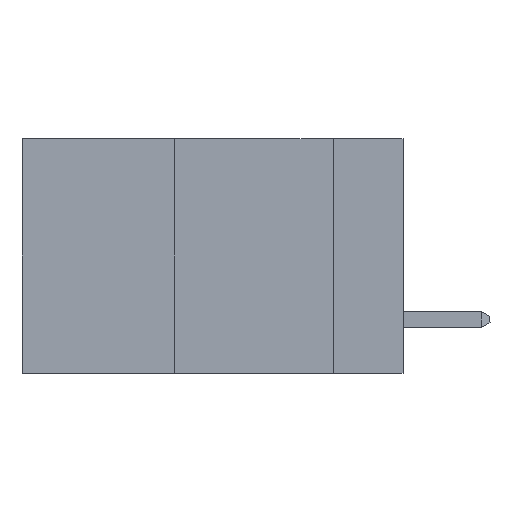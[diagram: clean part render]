
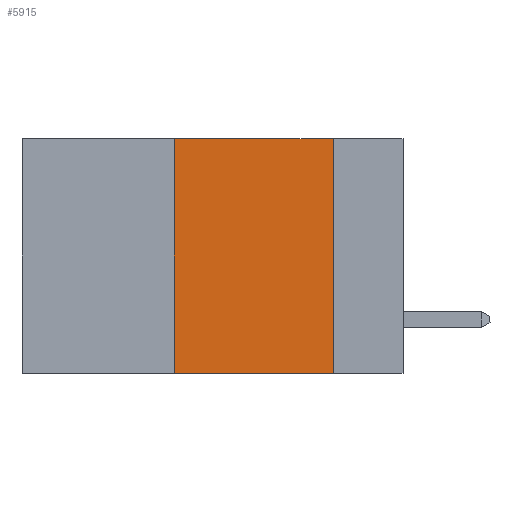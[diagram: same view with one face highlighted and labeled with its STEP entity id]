
A CAD part, left-side view. The second image highlights one B-rep face of the part: STEP entity #5915.
In plain terms, the highlighted planar face has unit normal (-1, 0, 0).
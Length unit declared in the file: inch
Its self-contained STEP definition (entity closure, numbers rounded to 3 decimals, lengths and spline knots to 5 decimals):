
#116 = DIRECTION ( 'NONE',  ( 1., 0., 0. ) ) ;
#634 = DIRECTION ( 'NONE',  ( 0., -1., 0. ) ) ;
#686 = VERTEX_POINT ( 'NONE', #8401 ) ;
#2073 = CARTESIAN_POINT ( 'NONE',  ( 0., 0.36, 0. ) ) ;
#2184 = EDGE_LOOP ( 'NONE', ( #16346, #13541, #3752, #4195 ) ) ;
#2306 = VECTOR ( 'NONE', #9709, 39.37008 ) ;
#2707 = CARTESIAN_POINT ( 'NONE',  ( 0., 0.11, 0. ) ) ;
#2923 = CARTESIAN_POINT ( 'NONE',  ( 0., 0.36, -0.37 ) ) ;
#3752 = ORIENTED_EDGE ( 'NONE', *, *, #6688, .F. ) ;
#4115 = VERTEX_POINT ( 'NONE', #15952 ) ;
#4149 = VECTOR ( 'NONE', #634, 39.37008 ) ;
#4195 = ORIENTED_EDGE ( 'NONE', *, *, #15907, .T. ) ;
#4337 = LINE ( 'NONE', #2073, #14973 ) ;
#4413 = PLANE ( 'NONE',  #9987 ) ;
#5442 = VECTOR ( 'NONE', #15236, 39.37008 ) ;
#5915 = ADVANCED_FACE ( 'NONE', ( #5943 ), #4413, .F. ) ;
#5943 = FACE_OUTER_BOUND ( 'NONE', #2184, .T. ) ;
#6688 = EDGE_CURVE ( 'NONE', #10595, #4115, #4337, .T. ) ;
#6973 = CARTESIAN_POINT ( 'NONE',  ( 0., 0.6, 0. ) ) ;
#8401 = CARTESIAN_POINT ( 'NONE',  ( 0., 0.11, 0. ) ) ;
#8651 = CARTESIAN_POINT ( 'NONE',  ( 0., 0.6, 0. ) ) ;
#9142 = LINE ( 'NONE', #6973, #5442 ) ;
#9709 = DIRECTION ( 'NONE',  ( 0., 0., -1. ) ) ;
#9773 = LINE ( 'NONE', #2707, #2306 ) ;
#9946 = CARTESIAN_POINT ( 'NONE',  ( 0., 0.11, -0.37 ) ) ;
#9987 = AXIS2_PLACEMENT_3D ( 'NONE', #8651, #116, #10019 ) ;
#10019 = DIRECTION ( 'NONE',  ( 0., 0., -1. ) ) ;
#10476 = DIRECTION ( 'NONE',  ( 0., 0., 1. ) ) ;
#10480 = CARTESIAN_POINT ( 'NONE',  ( 0., 0.6, -0.37 ) ) ;
#10595 = VERTEX_POINT ( 'NONE', #2923 ) ;
#11546 = LINE ( 'NONE', #10480, #4149 ) ;
#11784 = EDGE_CURVE ( 'NONE', #4115, #686, #9142, .T. ) ;
#13541 = ORIENTED_EDGE ( 'NONE', *, *, #11784, .F. ) ;
#14973 = VECTOR ( 'NONE', #10476, 39.37008 ) ;
#15236 = DIRECTION ( 'NONE',  ( 0., -1., 0. ) ) ;
#15633 = VERTEX_POINT ( 'NONE', #9946 ) ;
#15907 = EDGE_CURVE ( 'NONE', #10595, #15633, #11546, .T. ) ;
#15952 = CARTESIAN_POINT ( 'NONE',  ( 0., 0.36, 0. ) ) ;
#16346 = ORIENTED_EDGE ( 'NONE', *, *, #18097, .F. ) ;
#18097 = EDGE_CURVE ( 'NONE', #686, #15633, #9773, .T. ) ;
